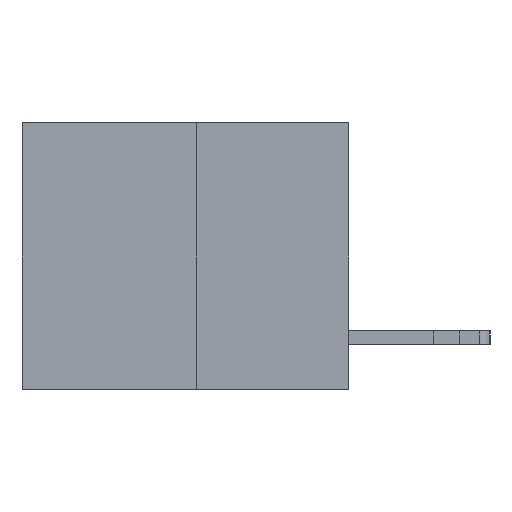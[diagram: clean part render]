
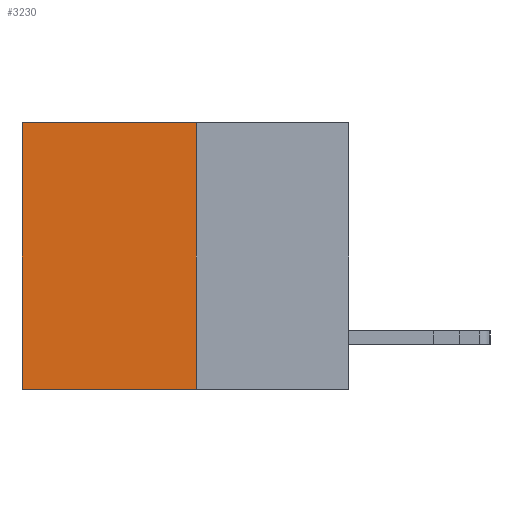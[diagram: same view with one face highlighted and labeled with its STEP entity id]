
A CAD part, left-side view. The second image highlights one B-rep face of the part: STEP entity #3230.
In plain terms, the highlighted planar face has unit normal (-1, 0, 0).
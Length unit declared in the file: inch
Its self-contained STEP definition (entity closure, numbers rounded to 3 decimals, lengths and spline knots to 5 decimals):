
#11 = LINE ( 'NONE', #3825, #5037 ) ;
#539 = DIRECTION ( 'NONE',  ( 1., 0., 0. ) ) ;
#767 = LINE ( 'NONE', #2761, #11198 ) ;
#1076 = ORIENTED_EDGE ( 'NONE', *, *, #2767, .T. ) ;
#1737 = DIRECTION ( 'NONE',  ( 0., 0., -1. ) ) ;
#2481 = DIRECTION ( 'NONE',  ( 0., 0., -1. ) ) ;
#2761 = CARTESIAN_POINT ( 'NONE',  ( 0.3165, 0.6, -0.49 ) ) ;
#2767 = EDGE_CURVE ( 'NONE', #5678, #2880, #767, .T. ) ;
#2880 = VERTEX_POINT ( 'NONE', #11993 ) ;
#3096 = AXIS2_PLACEMENT_3D ( 'NONE', #8557, #539, #2481 ) ;
#3230 = ADVANCED_FACE ( 'NONE', ( #4834 ), #12493, .F. ) ;
#3496 = VERTEX_POINT ( 'NONE', #6254 ) ;
#3577 = DIRECTION ( 'NONE',  ( 0., 1., 0. ) ) ;
#3825 = CARTESIAN_POINT ( 'NONE',  ( 0.3165, 0.28, -0.49 ) ) ;
#4834 = FACE_OUTER_BOUND ( 'NONE', #6705, .T. ) ;
#5037 = VECTOR ( 'NONE', #10802, 39.37008 ) ;
#5414 = ORIENTED_EDGE ( 'NONE', *, *, #9919, .F. ) ;
#5678 = VERTEX_POINT ( 'NONE', #12501 ) ;
#6254 = CARTESIAN_POINT ( 'NONE',  ( 0.3165, 0.28, 0. ) ) ;
#6521 = DIRECTION ( 'NONE',  ( 0., 0., -1. ) ) ;
#6538 = LINE ( 'NONE', #7441, #11921 ) ;
#6705 = EDGE_LOOP ( 'NONE', ( #1076, #5414, #11643, #10161 ) ) ;
#7013 = VERTEX_POINT ( 'NONE', #10120 ) ;
#7441 = CARTESIAN_POINT ( 'NONE',  ( 0.3165, 0.28, -0.49 ) ) ;
#8460 = VECTOR ( 'NONE', #3577, 39.37008 ) ;
#8531 = CARTESIAN_POINT ( 'NONE',  ( 0.3165, 0.28, 0. ) ) ;
#8557 = CARTESIAN_POINT ( 'NONE',  ( 0.3165, 0.28, -0.49 ) ) ;
#8642 = EDGE_CURVE ( 'NONE', #3496, #7013, #6538, .T. ) ;
#9919 = EDGE_CURVE ( 'NONE', #7013, #2880, #11, .T. ) ;
#10120 = CARTESIAN_POINT ( 'NONE',  ( 0.3165, 0.28, -0.49 ) ) ;
#10161 = ORIENTED_EDGE ( 'NONE', *, *, #10995, .T. ) ;
#10802 = DIRECTION ( 'NONE',  ( 0., 1., 0. ) ) ;
#10995 = EDGE_CURVE ( 'NONE', #3496, #5678, #12765, .T. ) ;
#11198 = VECTOR ( 'NONE', #1737, 39.37008 ) ;
#11643 = ORIENTED_EDGE ( 'NONE', *, *, #8642, .F. ) ;
#11921 = VECTOR ( 'NONE', #6521, 39.37008 ) ;
#11993 = CARTESIAN_POINT ( 'NONE',  ( 0.3165, 0.6, -0.49 ) ) ;
#12493 = PLANE ( 'NONE',  #3096 ) ;
#12501 = CARTESIAN_POINT ( 'NONE',  ( 0.3165, 0.6, 0. ) ) ;
#12765 = LINE ( 'NONE', #8531, #8460 ) ;
